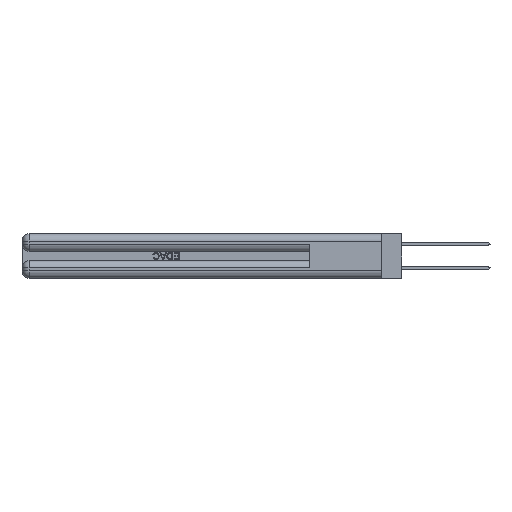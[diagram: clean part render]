
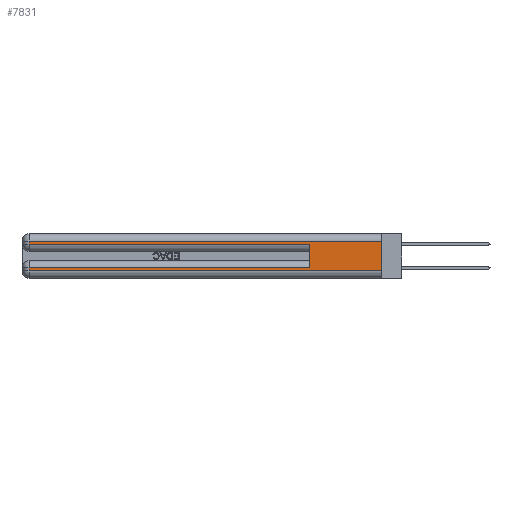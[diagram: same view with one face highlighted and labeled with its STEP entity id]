
A CAD part, left-side view. The second image highlights one B-rep face of the part: STEP entity #7831.
In plain terms, the highlighted planar face has unit normal (-1, 0, 0).
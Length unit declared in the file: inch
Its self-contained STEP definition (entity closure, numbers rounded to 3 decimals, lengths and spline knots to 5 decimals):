
#159 = DIRECTION ( 'NONE',  ( 0., 1., 0. ) ) ;
#292 = DIRECTION ( 'NONE',  ( 0., -1., 0. ) ) ;
#656 = CARTESIAN_POINT ( 'NONE',  ( 0., 2.94, 0.37 ) ) ;
#710 = VERTEX_POINT ( 'NONE', #21627 ) ;
#1890 = DIRECTION ( 'NONE',  ( 0., 0., 1. ) ) ;
#3236 = CARTESIAN_POINT ( 'NONE',  ( 0., 0.6, 0.285 ) ) ;
#5577 = EDGE_CURVE ( 'NONE', #9270, #710, #36822, .T. ) ;
#6994 = CARTESIAN_POINT ( 'NONE',  ( 0., 2.94, 0.31 ) ) ;
#7749 = VECTOR ( 'NONE', #27283, 39.37008 ) ;
#7831 = ADVANCED_FACE ( 'NONE', ( #11753 ), #28137, .F. ) ;
#9270 = VERTEX_POINT ( 'NONE', #6994 ) ;
#10595 = ORIENTED_EDGE ( 'NONE', *, *, #19111, .T. ) ;
#11753 = FACE_OUTER_BOUND ( 'NONE', #41981, .T. ) ;
#12006 = CARTESIAN_POINT ( 'NONE',  ( 0., 0., 0.37 ) ) ;
#12141 = LINE ( 'NONE', #22295, #21087 ) ;
#12637 = VECTOR ( 'NONE', #159, 39.37008 ) ;
#13027 = DIRECTION ( 'NONE',  ( 0., 0., -1. ) ) ;
#13129 = EDGE_CURVE ( 'NONE', #40421, #13982, #25169, .T. ) ;
#13910 = VECTOR ( 'NONE', #292, 39.37008 ) ;
#13982 = VERTEX_POINT ( 'NONE', #20228 ) ;
#14016 = LINE ( 'NONE', #47393, #34198 ) ;
#15623 = CARTESIAN_POINT ( 'NONE',  ( 0., 2.94, 0.085 ) ) ;
#16399 = VERTEX_POINT ( 'NONE', #41881 ) ;
#16931 = ORIENTED_EDGE ( 'NONE', *, *, #36427, .T. ) ;
#17962 = EDGE_CURVE ( 'NONE', #37877, #21329, #14016, .T. ) ;
#18738 = VECTOR ( 'NONE', #19930, 39.37008 ) ;
#19111 = EDGE_CURVE ( 'NONE', #710, #21329, #38961, .T. ) ;
#19181 = CARTESIAN_POINT ( 'NONE',  ( 0., 0., 0.085 ) ) ;
#19930 = DIRECTION ( 'NONE',  ( 0., 1., 0. ) ) ;
#20047 = ORIENTED_EDGE ( 'NONE', *, *, #17962, .F. ) ;
#20228 = CARTESIAN_POINT ( 'NONE',  ( 0., 0., 0.06 ) ) ;
#20502 = ORIENTED_EDGE ( 'NONE', *, *, #29128, .F. ) ;
#20611 = AXIS2_PLACEMENT_3D ( 'NONE', #46989, #35743, #13027 ) ;
#21087 = VECTOR ( 'NONE', #26766, 39.37008 ) ;
#21329 = VERTEX_POINT ( 'NONE', #3236 ) ;
#21627 = CARTESIAN_POINT ( 'NONE',  ( 0., 2.94, 0.285 ) ) ;
#22295 = CARTESIAN_POINT ( 'NONE',  ( 0., 2.94, 0.37 ) ) ;
#23055 = CARTESIAN_POINT ( 'NONE',  ( 0., 2.94, 0.06 ) ) ;
#23928 = LINE ( 'NONE', #19181, #12637 ) ;
#24853 = ORIENTED_EDGE ( 'NONE', *, *, #13129, .T. ) ;
#25169 = LINE ( 'NONE', #38171, #13910 ) ;
#26766 = DIRECTION ( 'NONE',  ( 0., 0., -1. ) ) ;
#27005 = CARTESIAN_POINT ( 'NONE',  ( 0., 0., 0.285 ) ) ;
#27283 = DIRECTION ( 'NONE',  ( 0., 0., -1. ) ) ;
#28137 = PLANE ( 'NONE',  #20611 ) ;
#28927 = VECTOR ( 'NONE', #38423, 39.37008 ) ;
#29128 = EDGE_CURVE ( 'NONE', #16399, #13982, #42643, .T. ) ;
#30011 = LINE ( 'NONE', #42546, #18738 ) ;
#31065 = ORIENTED_EDGE ( 'NONE', *, *, #35409, .T. ) ;
#32151 = VERTEX_POINT ( 'NONE', #15623 ) ;
#34198 = VECTOR ( 'NONE', #1890, 39.37008 ) ;
#34620 = EDGE_CURVE ( 'NONE', #32151, #40421, #12141, .T. ) ;
#35409 = EDGE_CURVE ( 'NONE', #16399, #9270, #30011, .T. ) ;
#35743 = DIRECTION ( 'NONE',  ( 1., 0., 0. ) ) ;
#36427 = EDGE_CURVE ( 'NONE', #37877, #32151, #23928, .T. ) ;
#36822 = LINE ( 'NONE', #656, #7749 ) ;
#37688 = ORIENTED_EDGE ( 'NONE', *, *, #34620, .T. ) ;
#37877 = VERTEX_POINT ( 'NONE', #47000 ) ;
#38171 = CARTESIAN_POINT ( 'NONE',  ( 0., 0., 0.06 ) ) ;
#38423 = DIRECTION ( 'NONE',  ( 0., -1., 0. ) ) ;
#38961 = LINE ( 'NONE', #27005, #28927 ) ;
#40277 = VECTOR ( 'NONE', #46467, 39.37008 ) ;
#40421 = VERTEX_POINT ( 'NONE', #23055 ) ;
#41881 = CARTESIAN_POINT ( 'NONE',  ( 0., 0., 0.31 ) ) ;
#41981 = EDGE_LOOP ( 'NONE', ( #20502, #31065, #42337, #10595, #20047, #16931, #37688, #24853 ) ) ;
#42337 = ORIENTED_EDGE ( 'NONE', *, *, #5577, .T. ) ;
#42546 = CARTESIAN_POINT ( 'NONE',  ( 0., 0., 0.31 ) ) ;
#42643 = LINE ( 'NONE', #12006, #40277 ) ;
#46467 = DIRECTION ( 'NONE',  ( 0., 0., -1. ) ) ;
#46989 = CARTESIAN_POINT ( 'NONE',  ( 0., 0., 0.37 ) ) ;
#47000 = CARTESIAN_POINT ( 'NONE',  ( 0., 0.6, 0.085 ) ) ;
#47393 = CARTESIAN_POINT ( 'NONE',  ( 0., 0.6, 0.145 ) ) ;
